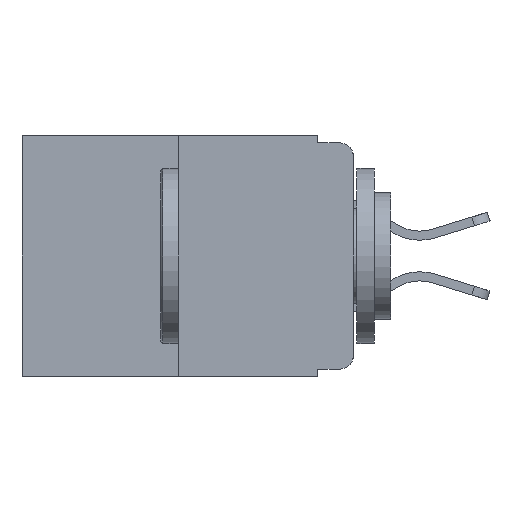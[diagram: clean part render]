
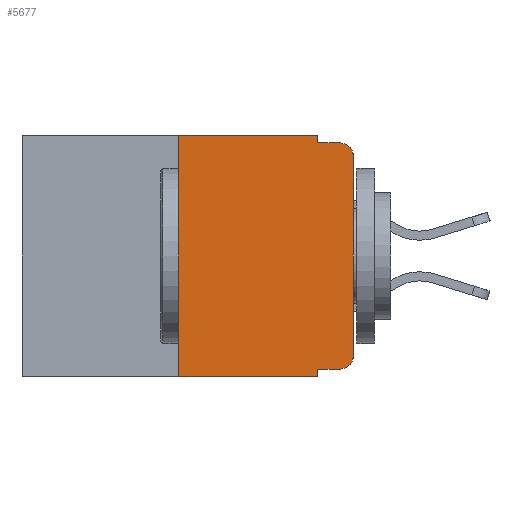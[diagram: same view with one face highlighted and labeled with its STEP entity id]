
A CAD part, left-side view. The second image highlights one B-rep face of the part: STEP entity #5677.
In plain terms, the highlighted planar face has unit normal (-1, 0, 0).
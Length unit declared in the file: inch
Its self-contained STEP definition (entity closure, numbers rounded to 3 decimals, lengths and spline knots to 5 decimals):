
#70 = VECTOR ( 'NONE', #1657, 39.37008 ) ;
#265 = DIRECTION ( 'NONE',  ( 0., 0., -1. ) ) ;
#356 = AXIS2_PLACEMENT_3D ( 'NONE', #925, #7698, #1963 ) ;
#479 = DIRECTION ( 'NONE',  ( 1., 0., 0. ) ) ;
#492 = CARTESIAN_POINT ( 'NONE',  ( 0., 0.25, 0. ) ) ;
#689 = LINE ( 'NONE', #11604, #3419 ) ;
#925 = CARTESIAN_POINT ( 'NONE',  ( 0., 0.02, -0.03 ) ) ;
#951 = VECTOR ( 'NONE', #1976, 39.37008 ) ;
#1057 = ORIENTED_EDGE ( 'NONE', *, *, #11590, .T. ) ;
#1136 = VERTEX_POINT ( 'NONE', #3493 ) ;
#1156 = EDGE_CURVE ( 'NONE', #7130, #6397, #7278, .T. ) ;
#1176 = EDGE_LOOP ( 'NONE', ( #5174, #1057, #10612, #2547, #9039, #5106, #5568, #11348, #10952, #4976 ) ) ;
#1262 = DIRECTION ( 'NONE',  ( -1., 0., 0. ) ) ;
#1392 = FACE_OUTER_BOUND ( 'NONE', #1176, .T. ) ;
#1408 = CARTESIAN_POINT ( 'NONE',  ( 0., 0.051, -0.343 ) ) ;
#1657 = DIRECTION ( 'NONE',  ( 0., 0., 1. ) ) ;
#1963 = DIRECTION ( 'NONE',  ( 0., 0., -1. ) ) ;
#1976 = DIRECTION ( 'NONE',  ( 0., -1., 0. ) ) ;
#2183 = CARTESIAN_POINT ( 'NONE',  ( 0., 0.051, -0.01 ) ) ;
#2547 = ORIENTED_EDGE ( 'NONE', *, *, #10417, .F. ) ;
#3226 = DIRECTION ( 'NONE',  ( 0., 0., -1. ) ) ;
#3419 = VECTOR ( 'NONE', #5446, 39.37008 ) ;
#3432 = CARTESIAN_POINT ( 'NONE',  ( 0., 0.02, -0.333 ) ) ;
#3493 = CARTESIAN_POINT ( 'NONE',  ( 0., 0., -0.03 ) ) ;
#3730 = VECTOR ( 'NONE', #3226, 39.37008 ) ;
#4643 = DIRECTION ( 'NONE',  ( 0., -1., 0. ) ) ;
#4659 = VECTOR ( 'NONE', #9953, 39.37008 ) ;
#4762 = AXIS2_PLACEMENT_3D ( 'NONE', #6415, #479, #7306 ) ;
#4838 = VECTOR ( 'NONE', #4643, 39.37008 ) ;
#4852 = CARTESIAN_POINT ( 'NONE',  ( 0., 0.051, 0. ) ) ;
#4959 = LINE ( 'NONE', #10792, #9436 ) ;
#4976 = ORIENTED_EDGE ( 'NONE', *, *, #8081, .T. ) ;
#5106 = ORIENTED_EDGE ( 'NONE', *, *, #9848, .F. ) ;
#5174 = ORIENTED_EDGE ( 'NONE', *, *, #12171, .T. ) ;
#5408 = CARTESIAN_POINT ( 'NONE',  ( 0., 0.25, -0.343 ) ) ;
#5446 = DIRECTION ( 'NONE',  ( 0., -1., 0. ) ) ;
#5568 = ORIENTED_EDGE ( 'NONE', *, *, #1156, .T. ) ;
#5609 = VERTEX_POINT ( 'NONE', #3432 ) ;
#5677 = ADVANCED_FACE ( 'NONE', ( #1392 ), #11655, .F. ) ;
#6248 = CARTESIAN_POINT ( 'NONE',  ( 0., 0.051, 0. ) ) ;
#6397 = VERTEX_POINT ( 'NONE', #1408 ) ;
#6415 = CARTESIAN_POINT ( 'NONE',  ( 0., 0.473, 0. ) ) ;
#6812 = VECTOR ( 'NONE', #265, 39.37008 ) ;
#7113 = CARTESIAN_POINT ( 'NONE',  ( 0., 0.02, -0.313 ) ) ;
#7130 = VERTEX_POINT ( 'NONE', #5408 ) ;
#7278 = LINE ( 'NONE', #10663, #4838 ) ;
#7306 = DIRECTION ( 'NONE',  ( 0., 0., -1. ) ) ;
#7462 = CARTESIAN_POINT ( 'NONE',  ( 0., 0., 0. ) ) ;
#7473 = VERTEX_POINT ( 'NONE', #4852 ) ;
#7647 = CARTESIAN_POINT ( 'NONE',  ( 0., 0., -0.313 ) ) ;
#7671 = VERTEX_POINT ( 'NONE', #7815 ) ;
#7698 = DIRECTION ( 'NONE',  ( -1., 0., 0. ) ) ;
#7815 = CARTESIAN_POINT ( 'NONE',  ( 0., 0.25, 0. ) ) ;
#7970 = CARTESIAN_POINT ( 'NONE',  ( 0., 0.051, -0.333 ) ) ;
#7993 = DIRECTION ( 'NONE',  ( 0., 0., -1. ) ) ;
#8073 = DIRECTION ( 'NONE',  ( 0., -1., 0. ) ) ;
#8081 = EDGE_CURVE ( 'NONE', #5609, #8468, #10285, .T. ) ;
#8468 = VERTEX_POINT ( 'NONE', #7647 ) ;
#8629 = LINE ( 'NONE', #9663, #3730 ) ;
#8670 = EDGE_CURVE ( 'NONE', #11234, #5609, #689, .T. ) ;
#8699 = CARTESIAN_POINT ( 'NONE',  ( 0., 0.02, -0.01 ) ) ;
#9039 = ORIENTED_EDGE ( 'NONE', *, *, #9776, .F. ) ;
#9262 = EDGE_CURVE ( 'NONE', #11234, #6397, #8629, .T. ) ;
#9436 = VECTOR ( 'NONE', #8073, 39.37008 ) ;
#9656 = LINE ( 'NONE', #7462, #70 ) ;
#9663 = CARTESIAN_POINT ( 'NONE',  ( 0., 0.051, 0. ) ) ;
#9776 = EDGE_CURVE ( 'NONE', #7671, #7473, #4959, .T. ) ;
#9848 = EDGE_CURVE ( 'NONE', #7130, #7671, #11469, .T. ) ;
#9953 = DIRECTION ( 'NONE',  ( 0., 0., 1. ) ) ;
#10285 = CIRCLE ( 'NONE', #11535, 0.02 ) ;
#10417 = EDGE_CURVE ( 'NONE', #7473, #11754, #11190, .T. ) ;
#10612 = ORIENTED_EDGE ( 'NONE', *, *, #11009, .F. ) ;
#10632 = LINE ( 'NONE', #12094, #951 ) ;
#10663 = CARTESIAN_POINT ( 'NONE',  ( 0., 0.473, -0.343 ) ) ;
#10792 = CARTESIAN_POINT ( 'NONE',  ( 0., 0.473, 0. ) ) ;
#10952 = ORIENTED_EDGE ( 'NONE', *, *, #8670, .T. ) ;
#11009 = EDGE_CURVE ( 'NONE', #11754, #11691, #10632, .T. ) ;
#11190 = LINE ( 'NONE', #6248, #6812 ) ;
#11234 = VERTEX_POINT ( 'NONE', #7970 ) ;
#11348 = ORIENTED_EDGE ( 'NONE', *, *, #9262, .F. ) ;
#11442 = CIRCLE ( 'NONE', #356, 0.02 ) ;
#11469 = LINE ( 'NONE', #492, #4659 ) ;
#11535 = AXIS2_PLACEMENT_3D ( 'NONE', #7113, #1262, #7993 ) ;
#11590 = EDGE_CURVE ( 'NONE', #1136, #11691, #11442, .T. ) ;
#11604 = CARTESIAN_POINT ( 'NONE',  ( 0., 0.051, -0.333 ) ) ;
#11655 = PLANE ( 'NONE',  #4762 ) ;
#11691 = VERTEX_POINT ( 'NONE', #8699 ) ;
#11754 = VERTEX_POINT ( 'NONE', #2183 ) ;
#12094 = CARTESIAN_POINT ( 'NONE',  ( 0., 0.051, -0.01 ) ) ;
#12171 = EDGE_CURVE ( 'NONE', #8468, #1136, #9656, .T. ) ;
